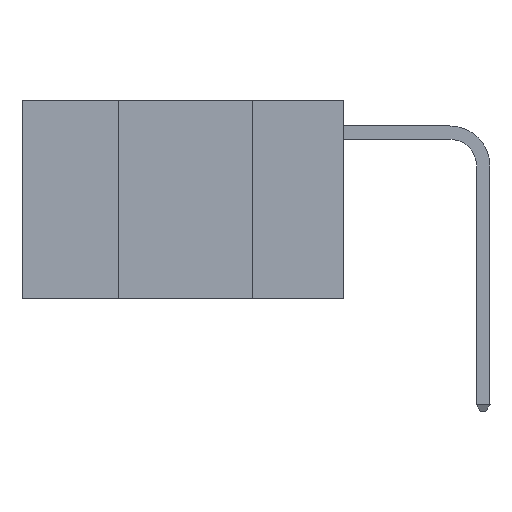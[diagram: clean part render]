
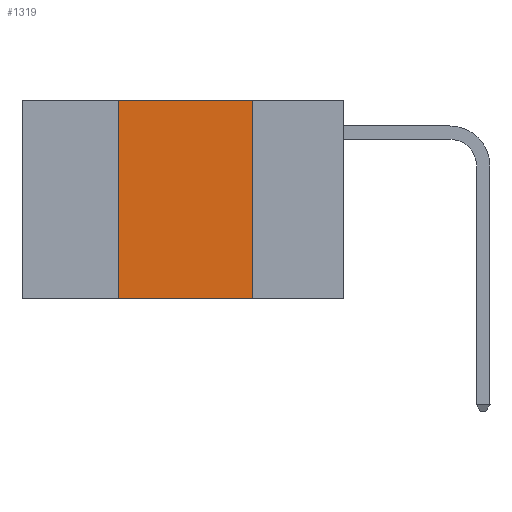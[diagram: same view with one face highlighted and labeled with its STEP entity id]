
A CAD part, left-side view. The second image highlights one B-rep face of the part: STEP entity #1319.
In plain terms, the highlighted planar face has unit normal (-1, 0, 0).
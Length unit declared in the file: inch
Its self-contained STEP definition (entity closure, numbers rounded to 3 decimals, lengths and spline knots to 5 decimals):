
#340 = CARTESIAN_POINT ( 'NONE',  ( 0., 0.42, 0. ) ) ;
#470 = ORIENTED_EDGE ( 'NONE', *, *, #1128, .T. ) ;
#541 = EDGE_CURVE ( 'NONE', #8833, #8578, #1908, .T. ) ;
#786 = EDGE_CURVE ( 'NONE', #8578, #9808, #3308, .T. ) ;
#853 = EDGE_CURVE ( 'NONE', #8051, #8833, #1396, .T. ) ;
#928 = CARTESIAN_POINT ( 'NONE',  ( 0., 0.17, -0.37 ) ) ;
#1128 = EDGE_CURVE ( 'NONE', #8051, #9808, #9227, .T. ) ;
#1319 = ADVANCED_FACE ( 'NONE', ( #3449 ), #8886, .F. ) ;
#1396 = LINE ( 'NONE', #3642, #1586 ) ;
#1586 = VECTOR ( 'NONE', #3779, 39.37008 ) ;
#1908 = LINE ( 'NONE', #3898, #1969 ) ;
#1969 = VECTOR ( 'NONE', #12247, 39.37008 ) ;
#3190 = VECTOR ( 'NONE', #7863, 39.37008 ) ;
#3308 = LINE ( 'NONE', #7861, #3190 ) ;
#3449 = FACE_OUTER_BOUND ( 'NONE', #11272, .T. ) ;
#3642 = CARTESIAN_POINT ( 'NONE',  ( 0., 0.42, 0. ) ) ;
#3779 = DIRECTION ( 'NONE',  ( 0., 0., 1. ) ) ;
#3898 = CARTESIAN_POINT ( 'NONE',  ( 0., 0.6, 0. ) ) ;
#5523 = CARTESIAN_POINT ( 'NONE',  ( 0., 0.42, -0.37 ) ) ;
#7861 = CARTESIAN_POINT ( 'NONE',  ( 0., 0.17, 0. ) ) ;
#7863 = DIRECTION ( 'NONE',  ( 0., 0., -1. ) ) ;
#8051 = VERTEX_POINT ( 'NONE', #5523 ) ;
#8172 = CARTESIAN_POINT ( 'NONE',  ( 0., 0.17, 0. ) ) ;
#8416 = VECTOR ( 'NONE', #11232, 39.37008 ) ;
#8578 = VERTEX_POINT ( 'NONE', #8172 ) ;
#8833 = VERTEX_POINT ( 'NONE', #340 ) ;
#8854 = DIRECTION ( 'NONE',  ( 0., 0., -1. ) ) ;
#8858 = DIRECTION ( 'NONE',  ( 1., 0., 0. ) ) ;
#8886 = PLANE ( 'NONE',  #11370 ) ;
#8982 = CARTESIAN_POINT ( 'NONE',  ( 0., 0.6, 0. ) ) ;
#9227 = LINE ( 'NONE', #11412, #8416 ) ;
#9808 = VERTEX_POINT ( 'NONE', #928 ) ;
#10573 = ORIENTED_EDGE ( 'NONE', *, *, #786, .F. ) ;
#11232 = DIRECTION ( 'NONE',  ( 0., -1., 0. ) ) ;
#11272 = EDGE_LOOP ( 'NONE', ( #10573, #12002, #12872, #470 ) ) ;
#11370 = AXIS2_PLACEMENT_3D ( 'NONE', #8982, #8858, #8854 ) ;
#11412 = CARTESIAN_POINT ( 'NONE',  ( 0., 0.6, -0.37 ) ) ;
#12002 = ORIENTED_EDGE ( 'NONE', *, *, #541, .F. ) ;
#12247 = DIRECTION ( 'NONE',  ( 0., -1., 0. ) ) ;
#12872 = ORIENTED_EDGE ( 'NONE', *, *, #853, .F. ) ;
